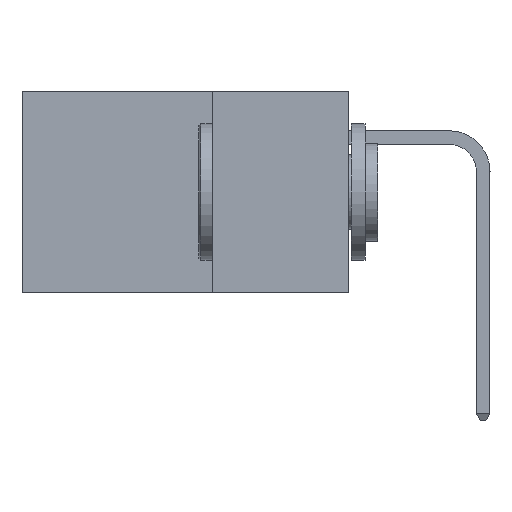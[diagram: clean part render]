
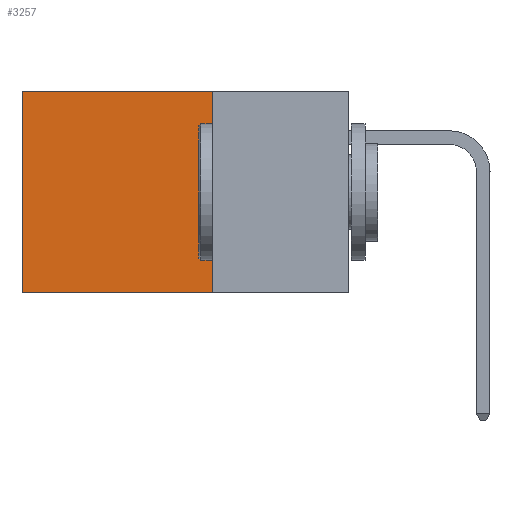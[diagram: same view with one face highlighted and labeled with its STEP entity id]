
A CAD part, left-side view. The second image highlights one B-rep face of the part: STEP entity #3257.
In plain terms, the highlighted planar face has unit normal (-1, 0, 0).
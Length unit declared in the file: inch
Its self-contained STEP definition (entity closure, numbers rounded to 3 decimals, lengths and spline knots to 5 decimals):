
#3166 = VERTEX_POINT ( 'NONE', #15429 ) ;
#3257 = ADVANCED_FACE ( 'NONE', ( #13203 ), #4316, .F. ) ;
#4308 = LINE ( 'NONE', #28992, #43839 ) ;
#4316 = PLANE ( 'NONE',  #6722 ) ;
#4925 = EDGE_LOOP ( 'NONE', ( #11572, #11479, #21437, #26735 ) ) ;
#6073 = DIRECTION ( 'NONE',  ( 0., 0., -1. ) ) ;
#6722 = AXIS2_PLACEMENT_3D ( 'NONE', #34980, #12070, #38831 ) ;
#7610 = VECTOR ( 'NONE', #45648, 39.37008 ) ;
#11430 = CARTESIAN_POINT ( 'NONE',  ( 0.2875, 0.25, 0. ) ) ;
#11479 = ORIENTED_EDGE ( 'NONE', *, *, #25025, .F. ) ;
#11572 = ORIENTED_EDGE ( 'NONE', *, *, #15659, .T. ) ;
#12070 = DIRECTION ( 'NONE',  ( 1., 0., 0. ) ) ;
#13203 = FACE_OUTER_BOUND ( 'NONE', #4925, .T. ) ;
#15388 = LINE ( 'NONE', #11430, #7610 ) ;
#15429 = CARTESIAN_POINT ( 'NONE',  ( 0.2875, 0.25, 0. ) ) ;
#15659 = EDGE_CURVE ( 'NONE', #44015, #45585, #20508, .T. ) ;
#20508 = LINE ( 'NONE', #40546, #30724 ) ;
#21437 = ORIENTED_EDGE ( 'NONE', *, *, #27266, .F. ) ;
#21503 = DIRECTION ( 'NONE',  ( 0., 0., -1. ) ) ;
#22979 = DIRECTION ( 'NONE',  ( 0., 1., 0. ) ) ;
#25025 = EDGE_CURVE ( 'NONE', #47411, #45585, #28593, .T. ) ;
#26735 = ORIENTED_EDGE ( 'NONE', *, *, #49182, .T. ) ;
#27266 = EDGE_CURVE ( 'NONE', #3166, #47411, #4308, .T. ) ;
#28593 = LINE ( 'NONE', #45842, #48887 ) ;
#28992 = CARTESIAN_POINT ( 'NONE',  ( 0.2875, 0.25, 0. ) ) ;
#30724 = VECTOR ( 'NONE', #21503, 39.37008 ) ;
#32563 = CARTESIAN_POINT ( 'NONE',  ( 0.2875, 0.6, -0.37 ) ) ;
#34980 = CARTESIAN_POINT ( 'NONE',  ( 0.2875, 0.25, 0. ) ) ;
#38831 = DIRECTION ( 'NONE',  ( 0., 0., -1. ) ) ;
#40546 = CARTESIAN_POINT ( 'NONE',  ( 0.2875, 0.6, 0. ) ) ;
#43839 = VECTOR ( 'NONE', #6073, 39.37008 ) ;
#44015 = VERTEX_POINT ( 'NONE', #49641 ) ;
#45585 = VERTEX_POINT ( 'NONE', #32563 ) ;
#45648 = DIRECTION ( 'NONE',  ( 0., 1., 0. ) ) ;
#45842 = CARTESIAN_POINT ( 'NONE',  ( 0.2875, 0.25, -0.37 ) ) ;
#46785 = CARTESIAN_POINT ( 'NONE',  ( 0.2875, 0.25, -0.37 ) ) ;
#47411 = VERTEX_POINT ( 'NONE', #46785 ) ;
#48887 = VECTOR ( 'NONE', #22979, 39.37008 ) ;
#49182 = EDGE_CURVE ( 'NONE', #3166, #44015, #15388, .T. ) ;
#49641 = CARTESIAN_POINT ( 'NONE',  ( 0.2875, 0.6, 0. ) ) ;
